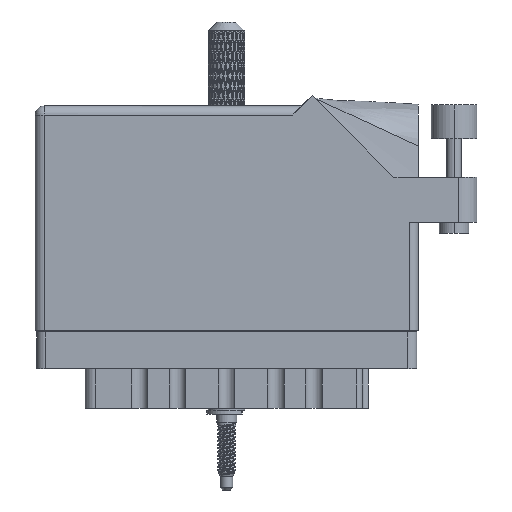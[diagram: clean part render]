
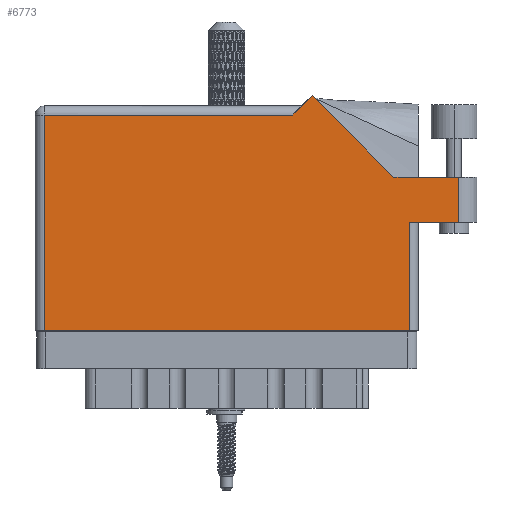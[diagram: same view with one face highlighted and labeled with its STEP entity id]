
A CAD part, front view. The second image highlights one B-rep face of the part: STEP entity #6773.
In plain terms, the highlighted face is planar.
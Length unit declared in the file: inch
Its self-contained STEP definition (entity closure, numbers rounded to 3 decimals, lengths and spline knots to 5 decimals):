
#1247 = VERTEX_POINT ( 'NONE', #4817 ) ;
#3602 = EDGE_LOOP ( 'NONE', ( #109066, #110886, #30755, #19667, #109566, #5952, #99546, #70630, #39380 ) ) ;
#4262 = CARTESIAN_POINT ( 'NONE',  ( 2.55, 0., 0. ) ) ;
#4817 = CARTESIAN_POINT ( 'NONE',  ( 1.88971, 1.60071, 0. ) ) ;
#5160 = CARTESIAN_POINT ( 'NONE',  ( 3.012, 1.044, 0. ) ) ;
#5952 = ORIENTED_EDGE ( 'NONE', *, *, #22280, .T. ) ;
#6208 = LINE ( 'NONE', #71207, #63047 ) ;
#6439 = CARTESIAN_POINT ( 'NONE',  ( 1.757, 1.468, 0. ) ) ;
#6773 = ADVANCED_FACE ( 'NONE', ( #21621 ), #63359, .F. ) ;
#6831 = DIRECTION ( 'NONE',  ( 1., 0., 0. ) ) ;
#9656 = CARTESIAN_POINT ( 'NONE',  ( 2.887, 1.044, 0. ) ) ;
#9947 = VECTOR ( 'NONE', #96149, 39.37008 ) ;
#10719 = EDGE_CURVE ( 'NONE', #76280, #53259, #109863, .T. ) ;
#12130 = VERTEX_POINT ( 'NONE', #6439 ) ;
#19064 = CARTESIAN_POINT ( 'NONE',  ( 2.55, 0.737, 0. ) ) ;
#19667 = ORIENTED_EDGE ( 'NONE', *, *, #47007, .T. ) ;
#21621 = FACE_OUTER_BOUND ( 'NONE', #3602, .T. ) ;
#21643 = VECTOR ( 'NONE', #36148, 39.37008 ) ;
#22280 = EDGE_CURVE ( 'NONE', #12130, #114332, #104204, .T. ) ;
#26443 = VERTEX_POINT ( 'NONE', #19064 ) ;
#27184 = LINE ( 'NONE', #50649, #77170 ) ;
#28049 = DIRECTION ( 'NONE',  ( 0., 0., -1. ) ) ;
#30755 = ORIENTED_EDGE ( 'NONE', *, *, #95580, .T. ) ;
#32566 = VECTOR ( 'NONE', #6831, 39.37008 ) ;
#35816 = CARTESIAN_POINT ( 'NONE',  ( 0., 1.53, 0. ) ) ;
#36148 = DIRECTION ( 'NONE',  ( 1., 0., 0. ) ) ;
#36959 = DIRECTION ( 'NONE',  ( -1., 0., 0. ) ) ;
#37370 = DIRECTION ( 'NONE',  ( -0.707, 0.707, 0. ) ) ;
#39380 = ORIENTED_EDGE ( 'NONE', *, *, #56956, .T. ) ;
#41206 = CARTESIAN_POINT ( 'NONE',  ( 2.44642, 1.044, 0. ) ) ;
#42227 = CARTESIAN_POINT ( 'NONE',  ( 2.887, 0.737, 0. ) ) ;
#45295 = DIRECTION ( 'NONE',  ( 0., 1., 0. ) ) ;
#47007 = EDGE_CURVE ( 'NONE', #71465, #1247, #97160, .T. ) ;
#49317 = DIRECTION ( 'NONE',  ( -1., 0., 0. ) ) ;
#50649 = CARTESIAN_POINT ( 'NONE',  ( 0.062, 0., 0. ) ) ;
#52362 = VERTEX_POINT ( 'NONE', #4262 ) ;
#53259 = VERTEX_POINT ( 'NONE', #70303 ) ;
#54058 = DIRECTION ( 'NONE',  ( -0.707, -0.707, 0. ) ) ;
#56956 = EDGE_CURVE ( 'NONE', #52362, #26443, #102848, .T. ) ;
#59666 = DIRECTION ( 'NONE',  ( 0., 1., 0. ) ) ;
#60636 = CARTESIAN_POINT ( 'NONE',  ( 0., 1.468, 0. ) ) ;
#63047 = VECTOR ( 'NONE', #54058, 39.37008 ) ;
#63311 = CARTESIAN_POINT ( 'NONE',  ( 0.062, 1.468, 0. ) ) ;
#63359 = PLANE ( 'NONE',  #100343 ) ;
#67484 = LINE ( 'NONE', #97700, #21643 ) ;
#68142 = DIRECTION ( 'NONE',  ( 0., -1., 0. ) ) ;
#70303 = CARTESIAN_POINT ( 'NONE',  ( 2.887, 1.044, 0. ) ) ;
#70630 = ORIENTED_EDGE ( 'NONE', *, *, #82015, .T. ) ;
#71019 = VECTOR ( 'NONE', #45295, 39.37008 ) ;
#71207 = CARTESIAN_POINT ( 'NONE',  ( 1.819, 1.53, 0. ) ) ;
#71465 = VERTEX_POINT ( 'NONE', #41206 ) ;
#74349 = EDGE_CURVE ( 'NONE', #114332, #101936, #27184, .T. ) ;
#76280 = VERTEX_POINT ( 'NONE', #42227 ) ;
#76636 = EDGE_CURVE ( 'NONE', #1247, #12130, #6208, .T. ) ;
#77170 = VECTOR ( 'NONE', #68142, 39.37008 ) ;
#78178 = CARTESIAN_POINT ( 'NONE',  ( 0.062, 0., 0. ) ) ;
#79747 = LINE ( 'NONE', #86312, #32566 ) ;
#82015 = EDGE_CURVE ( 'NONE', #101936, #52362, #79747, .T. ) ;
#86312 = CARTESIAN_POINT ( 'NONE',  ( 0., 0., 0. ) ) ;
#91751 = VECTOR ( 'NONE', #59666, 39.37008 ) ;
#95580 = EDGE_CURVE ( 'NONE', #53259, #71465, #110785, .T. ) ;
#96149 = DIRECTION ( 'NONE',  ( -1., 0., 0. ) ) ;
#97160 = LINE ( 'NONE', #99687, #113903 ) ;
#97700 = CARTESIAN_POINT ( 'NONE',  ( 2.612, 0.737, 0. ) ) ;
#99546 = ORIENTED_EDGE ( 'NONE', *, *, #74349, .T. ) ;
#99687 = CARTESIAN_POINT ( 'NONE',  ( 2.44642, 1.044, 0. ) ) ;
#100343 = AXIS2_PLACEMENT_3D ( 'NONE', #35816, #28049, #36959 ) ;
#101936 = VERTEX_POINT ( 'NONE', #78178 ) ;
#102848 = LINE ( 'NONE', #112695, #91751 ) ;
#103869 = VECTOR ( 'NONE', #49317, 39.37008 ) ;
#104204 = LINE ( 'NONE', #60636, #9947 ) ;
#109066 = ORIENTED_EDGE ( 'NONE', *, *, #114251, .T. ) ;
#109566 = ORIENTED_EDGE ( 'NONE', *, *, #76636, .T. ) ;
#109863 = LINE ( 'NONE', #9656, #71019 ) ;
#110785 = LINE ( 'NONE', #5160, #103869 ) ;
#110886 = ORIENTED_EDGE ( 'NONE', *, *, #10719, .T. ) ;
#112695 = CARTESIAN_POINT ( 'NONE',  ( 2.55, 0.737, 0. ) ) ;
#113903 = VECTOR ( 'NONE', #37370, 39.37008 ) ;
#114251 = EDGE_CURVE ( 'NONE', #26443, #76280, #67484, .T. ) ;
#114332 = VERTEX_POINT ( 'NONE', #63311 ) ;
